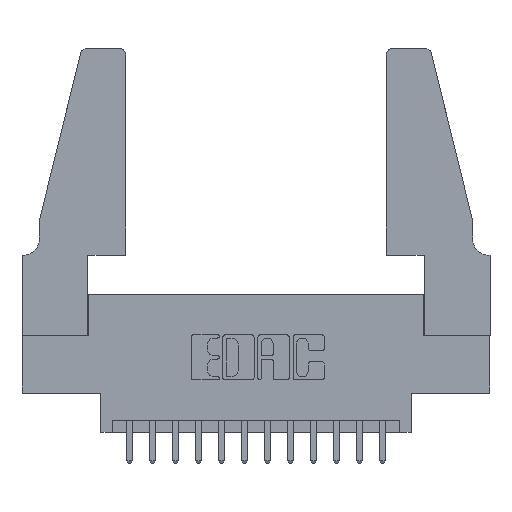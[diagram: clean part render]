
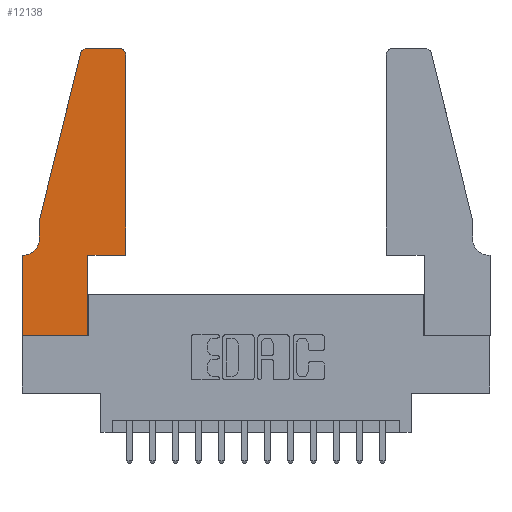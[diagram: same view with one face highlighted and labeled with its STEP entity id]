
A CAD part, top view. The second image highlights one B-rep face of the part: STEP entity #12138.
In plain terms, the highlighted planar face has unit normal (0, 0, 1).
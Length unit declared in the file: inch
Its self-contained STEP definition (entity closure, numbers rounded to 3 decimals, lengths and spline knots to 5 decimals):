
#75 = AXIS2_PLACEMENT_3D ( 'NONE', #7998, #484, #9188 ) ;
#206 = CARTESIAN_POINT ( 'NONE',  ( 0.2605, 1.25, 0.37 ) ) ;
#303 = CARTESIAN_POINT ( 'NONE',  ( 0.0755, 0.5, 0.37 ) ) ;
#484 = DIRECTION ( 'NONE',  ( 0., 0., -1. ) ) ;
#573 = CARTESIAN_POINT ( 'NONE',  ( 0.4505, 0.35, 0.37 ) ) ;
#584 = DIRECTION ( 'NONE',  ( 1., 0., 0. ) ) ;
#679 = ORIENTED_EDGE ( 'NONE', *, *, #3631, .T. ) ;
#733 = VERTEX_POINT ( 'NONE', #573 ) ;
#808 = CARTESIAN_POINT ( 'NONE',  ( 0.2865, 0.35, 0.37 ) ) ;
#1140 = VERTEX_POINT ( 'NONE', #15694 ) ;
#1202 = CARTESIAN_POINT ( 'NONE',  ( 0.0755, 0.5, 0.37 ) ) ;
#1315 = VERTEX_POINT ( 'NONE', #5627 ) ;
#1610 = CIRCLE ( 'NONE', #12501, 0.03 ) ;
#1726 = VECTOR ( 'NONE', #12488, 39.37008 ) ;
#1752 = ORIENTED_EDGE ( 'NONE', *, *, #14543, .T. ) ;
#2086 = AXIS2_PLACEMENT_3D ( 'NONE', #4335, #8084, #584 ) ;
#2729 = CARTESIAN_POINT ( 'NONE',  ( 0.0755, 0.35, 0.37 ) ) ;
#3030 = CARTESIAN_POINT ( 'NONE',  ( 0.4205, 1.22, 0.37 ) ) ;
#3036 = EDGE_CURVE ( 'NONE', #4720, #14737, #6279, .T. ) ;
#3047 = PLANE ( 'NONE',  #2086 ) ;
#3631 = EDGE_CURVE ( 'NONE', #11635, #5891, #8352, .T. ) ;
#3644 = CARTESIAN_POINT ( 'NONE',  ( 0.0755, 0.42, 0.37 ) ) ;
#3981 = ORIENTED_EDGE ( 'NONE', *, *, #7458, .T. ) ;
#4318 = DIRECTION ( 'NONE',  ( 1., 0., 0. ) ) ;
#4335 = CARTESIAN_POINT ( 'NONE',  ( 0., 0.35, 0.37 ) ) ;
#4339 = ORIENTED_EDGE ( 'NONE', *, *, #4474, .T. ) ;
#4343 = DIRECTION ( 'NONE',  ( 0., -1., 0. ) ) ;
#4474 = EDGE_CURVE ( 'NONE', #15245, #10026, #5599, .T. ) ;
#4528 = DIRECTION ( 'NONE',  ( 1., 0., 0. ) ) ;
#4685 = LINE ( 'NONE', #2729, #7226 ) ;
#4720 = VERTEX_POINT ( 'NONE', #3644 ) ;
#4785 = CARTESIAN_POINT ( 'NONE',  ( 0.4505, 0.35, 0.37 ) ) ;
#5082 = VERTEX_POINT ( 'NONE', #1202 ) ;
#5403 = ORIENTED_EDGE ( 'NONE', *, *, #12753, .T. ) ;
#5599 = LINE ( 'NONE', #10621, #11628 ) ;
#5627 = CARTESIAN_POINT ( 'NONE',  ( 0.25487, 1.22718, 0.37 ) ) ;
#5891 = VERTEX_POINT ( 'NONE', #11296 ) ;
#5924 = EDGE_CURVE ( 'NONE', #1315, #5082, #14597, .T. ) ;
#6000 = DIRECTION ( 'NONE',  ( 0., 0., 1. ) ) ;
#6136 = CARTESIAN_POINT ( 'NONE',  ( 0.0755, 0.5, 0.37 ) ) ;
#6279 = CIRCLE ( 'NONE', #75, 0.07 ) ;
#6618 = CARTESIAN_POINT ( 'NONE',  ( 0.2865, 0.35, 0.37 ) ) ;
#6635 = CARTESIAN_POINT ( 'NONE',  ( 0., 0., 0.37 ) ) ;
#6835 = ORIENTED_EDGE ( 'NONE', *, *, #6840, .T. ) ;
#6840 = EDGE_CURVE ( 'NONE', #5891, #1315, #1610, .T. ) ;
#6866 = CARTESIAN_POINT ( 'NONE',  ( 0.0055, 0.35, 0.37 ) ) ;
#6882 = EDGE_CURVE ( 'NONE', #13921, #733, #13082, .T. ) ;
#7012 = VECTOR ( 'NONE', #14496, 39.37008 ) ;
#7068 = CIRCLE ( 'NONE', #13256, 0.03 ) ;
#7226 = VECTOR ( 'NONE', #10134, 39.37008 ) ;
#7458 = EDGE_CURVE ( 'NONE', #10026, #13921, #15085, .T. ) ;
#7843 = EDGE_CURVE ( 'NONE', #733, #1140, #15072, .T. ) ;
#7865 = DIRECTION ( 'NONE',  ( 0., 1., 0. ) ) ;
#7998 = CARTESIAN_POINT ( 'NONE',  ( 0.0055, 0.42, 0.37 ) ) ;
#8084 = DIRECTION ( 'NONE',  ( 0., 0., 1. ) ) ;
#8352 = LINE ( 'NONE', #206, #1726 ) ;
#8997 = DIRECTION ( 'NONE',  ( -0.239, -0.971, 0. ) ) ;
#9057 = EDGE_CURVE ( 'NONE', #14792, #15245, #13010, .T. ) ;
#9188 = DIRECTION ( 'NONE',  ( -1., 0., 0. ) ) ;
#9407 = CARTESIAN_POINT ( 'NONE',  ( 0.4205, 1.25, 0.37 ) ) ;
#9833 = ORIENTED_EDGE ( 'NONE', *, *, #9986, .T. ) ;
#9945 = VECTOR ( 'NONE', #14413, 39.37008 ) ;
#9986 = EDGE_CURVE ( 'NONE', #5082, #4720, #12600, .T. ) ;
#10026 = VERTEX_POINT ( 'NONE', #13432 ) ;
#10134 = DIRECTION ( 'NONE',  ( -1., 0., 0. ) ) ;
#10621 = CARTESIAN_POINT ( 'NONE',  ( 0., 0., 0.37 ) ) ;
#10687 = DIRECTION ( 'NONE',  ( 0., 1., 0. ) ) ;
#11296 = CARTESIAN_POINT ( 'NONE',  ( 0.284, 1.25, 0.37 ) ) ;
#11390 = CARTESIAN_POINT ( 'NONE',  ( 0.4505, 0.35, 0.37 ) ) ;
#11588 = DIRECTION ( 'NONE',  ( 0., 0., 1. ) ) ;
#11628 = VECTOR ( 'NONE', #4528, 39.37008 ) ;
#11635 = VERTEX_POINT ( 'NONE', #9407 ) ;
#11746 = CARTESIAN_POINT ( 'NONE',  ( 0., 0.35, 0.37 ) ) ;
#11791 = VECTOR ( 'NONE', #8997, 39.37008 ) ;
#11909 = VECTOR ( 'NONE', #7865, 39.37008 ) ;
#12138 = ADVANCED_FACE ( 'NONE', ( #15264 ), #3047, .T. ) ;
#12290 = ORIENTED_EDGE ( 'NONE', *, *, #6882, .T. ) ;
#12443 = ORIENTED_EDGE ( 'NONE', *, *, #9057, .T. ) ;
#12488 = DIRECTION ( 'NONE',  ( -1., 0., 0. ) ) ;
#12501 = AXIS2_PLACEMENT_3D ( 'NONE', #13184, #6000, #14362 ) ;
#12538 = ORIENTED_EDGE ( 'NONE', *, *, #3036, .T. ) ;
#12557 = ORIENTED_EDGE ( 'NONE', *, *, #7843, .T. ) ;
#12600 = LINE ( 'NONE', #6136, #7012 ) ;
#12753 = EDGE_CURVE ( 'NONE', #1140, #11635, #7068, .T. ) ;
#12818 = CARTESIAN_POINT ( 'NONE',  ( 0., 0., 0.37 ) ) ;
#12953 = EDGE_LOOP ( 'NONE', ( #679, #6835, #13874, #9833, #12538, #1752, #12443, #4339, #3981, #12290, #12557, #5403 ) ) ;
#13010 = LINE ( 'NONE', #12818, #15785 ) ;
#13082 = LINE ( 'NONE', #4785, #9945 ) ;
#13184 = CARTESIAN_POINT ( 'NONE',  ( 0.284, 1.22, 0.37 ) ) ;
#13256 = AXIS2_PLACEMENT_3D ( 'NONE', #3030, #11588, #4318 ) ;
#13432 = CARTESIAN_POINT ( 'NONE',  ( 0.2865, 0., 0.37 ) ) ;
#13874 = ORIENTED_EDGE ( 'NONE', *, *, #5924, .T. ) ;
#13921 = VERTEX_POINT ( 'NONE', #6618 ) ;
#14362 = DIRECTION ( 'NONE',  ( 1., 0., 0. ) ) ;
#14413 = DIRECTION ( 'NONE',  ( 1., 0., 0. ) ) ;
#14496 = DIRECTION ( 'NONE',  ( 0., -1., 0. ) ) ;
#14543 = EDGE_CURVE ( 'NONE', #14737, #14792, #4685, .T. ) ;
#14597 = LINE ( 'NONE', #303, #11791 ) ;
#14734 = VECTOR ( 'NONE', #10687, 39.37008 ) ;
#14737 = VERTEX_POINT ( 'NONE', #6866 ) ;
#14792 = VERTEX_POINT ( 'NONE', #11746 ) ;
#15072 = LINE ( 'NONE', #11390, #11909 ) ;
#15085 = LINE ( 'NONE', #808, #14734 ) ;
#15245 = VERTEX_POINT ( 'NONE', #6635 ) ;
#15264 = FACE_OUTER_BOUND ( 'NONE', #12953, .T. ) ;
#15694 = CARTESIAN_POINT ( 'NONE',  ( 0.4505, 1.22, 0.37 ) ) ;
#15785 = VECTOR ( 'NONE', #4343, 39.37008 ) ;
